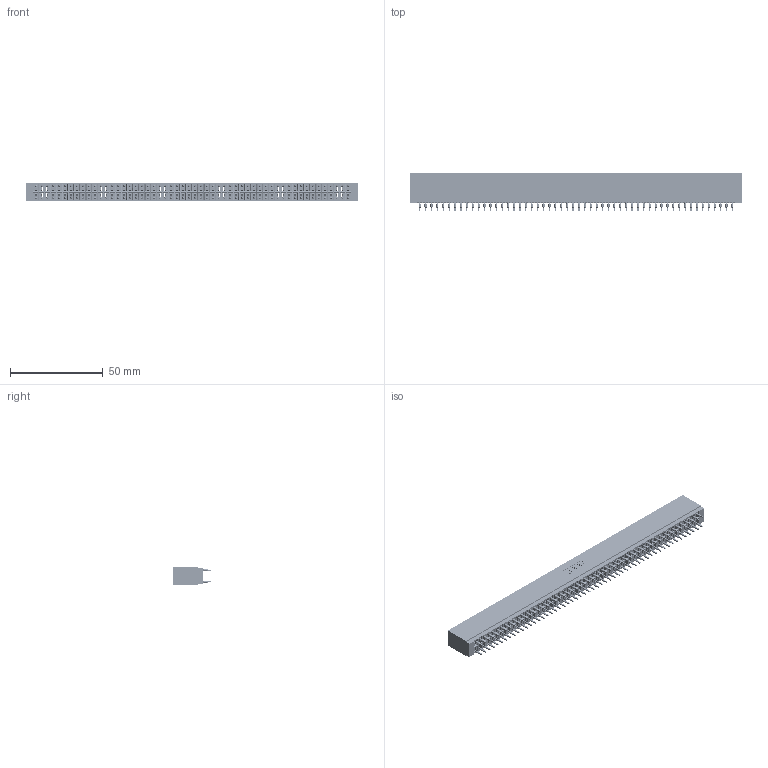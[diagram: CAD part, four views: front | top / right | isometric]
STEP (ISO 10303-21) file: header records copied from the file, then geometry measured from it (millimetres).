
FILE_DESCRIPTION (( 'STEP AP203' ), '1' );
FILE_NAME ('746-108-560-201.STEP', '2026-03-05T00:24:26', ( '' ), ( '' ), 'SwSTEP 2.0', 'SolidWorks 2023', '' );
FILE_SCHEMA (( 'CONFIG_CONTROL_DESIGN' ));
Length unit declared in the file: millimetre
Products named in the file (3): 746-108-560-201; 746 Part_.515 Slot Depth - 01; 746-292-001_560
Assembly tree (109 placements, depth 2):
  746-108-560-201
    746 Part_.515 Slot Depth - 01
    746-292-001_560  x108
Bounding box: 178.69 x 20.82 x 9.91 mm (x, y, z)
Volume: 19450.4 mm3; surface area: 33234.3 mm2
Topology: 109 solids, 109 shells, 10303 faces, 28667 edges, 18373 vertices
Faces by surface type: plane 5131, cylinder 2364, bspline 2160, torus 648
Entity records: 81824 total; most frequent: CARTESIAN_POINT 16159, ORIENTED_EDGE 14106, DIRECTION 11763, EDGE_CURVE 7053, LINE 6321, VECTOR 6321, VERTEX_POINT 4677, AXIS2_PLACEMENT_3D 2721
